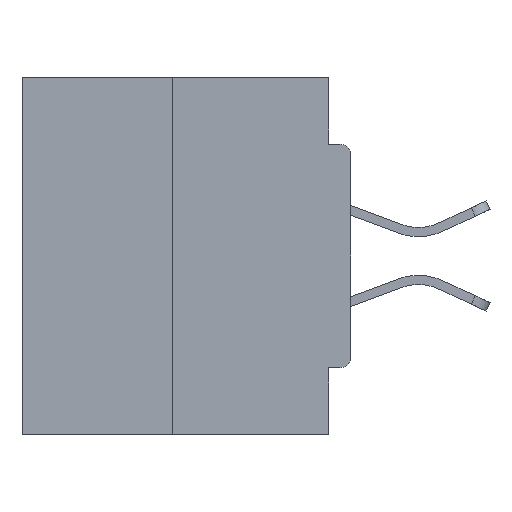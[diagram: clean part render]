
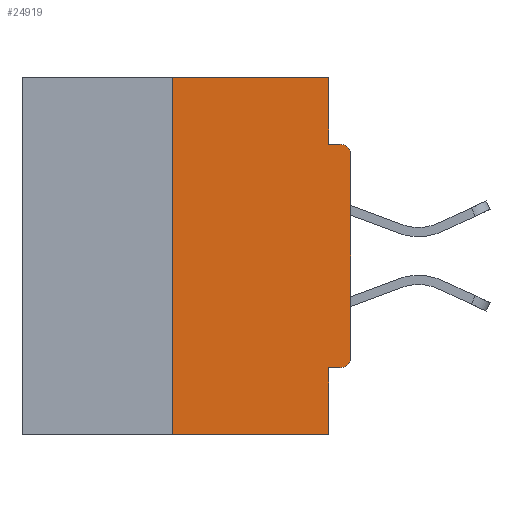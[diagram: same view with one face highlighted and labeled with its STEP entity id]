
A CAD part, left-side view. The second image highlights one B-rep face of the part: STEP entity #24919.
In plain terms, the highlighted planar face has unit normal (-1, 0, 0).
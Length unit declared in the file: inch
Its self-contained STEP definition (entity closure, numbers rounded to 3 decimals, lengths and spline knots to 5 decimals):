
#801 = EDGE_CURVE ( 'NONE', #25717, #2576, #8474, .T. ) ;
#1323 = LINE ( 'NONE', #11210, #20976 ) ;
#2336 = VERTEX_POINT ( 'NONE', #19962 ) ;
#2545 = CARTESIAN_POINT ( 'NONE',  ( 0., 0., 0. ) ) ;
#2576 = VERTEX_POINT ( 'NONE', #5639 ) ;
#3065 = AXIS2_PLACEMENT_3D ( 'NONE', #5719, #31607, #26658 ) ;
#4109 = DIRECTION ( 'NONE',  ( 0., 1., 0. ) ) ;
#4173 = VECTOR ( 'NONE', #32943, 39.37008 ) ;
#4766 = EDGE_CURVE ( 'NONE', #33345, #22715, #27988, .T. ) ;
#4966 = EDGE_CURVE ( 'NONE', #25717, #9873, #32548, .T. ) ;
#5000 = DIRECTION ( 'NONE',  ( 0., -1., 0. ) ) ;
#5095 = DIRECTION ( 'NONE',  ( 0., 0., 1. ) ) ;
#5639 = CARTESIAN_POINT ( 'NONE',  ( 0., 0., -0.3915 ) ) ;
#5697 = PLANE ( 'NONE',  #27454 ) ;
#5719 = CARTESIAN_POINT ( 'NONE',  ( 0., 0.015, -0.3915 ) ) ;
#5952 = VERTEX_POINT ( 'NONE', #12045 ) ;
#6232 = VECTOR ( 'NONE', #33441, 39.37008 ) ;
#7066 = LINE ( 'NONE', #14734, #4173 ) ;
#7301 = AXIS2_PLACEMENT_3D ( 'NONE', #10807, #23430, #23251 ) ;
#7408 = CARTESIAN_POINT ( 'NONE',  ( 0., 0.015, -0.0935 ) ) ;
#7714 = LINE ( 'NONE', #21163, #23079 ) ;
#8062 = EDGE_CURVE ( 'NONE', #2576, #2336, #18870, .T. ) ;
#8221 = DIRECTION ( 'NONE',  ( 0., 0., 1. ) ) ;
#8474 = CIRCLE ( 'NONE', #3065, 0.015 ) ;
#8845 = CARTESIAN_POINT ( 'NONE',  ( 0., 0.031, 0. ) ) ;
#9762 = LINE ( 'NONE', #28315, #9918 ) ;
#9873 = VERTEX_POINT ( 'NONE', #13396 ) ;
#9918 = VECTOR ( 'NONE', #12482, 39.37008 ) ;
#9944 = CARTESIAN_POINT ( 'NONE',  ( 0., 0.46, -0.5 ) ) ;
#10517 = EDGE_CURVE ( 'NONE', #5952, #23586, #12670, .T. ) ;
#10557 = CIRCLE ( 'NONE', #7301, 0.015 ) ;
#10807 = CARTESIAN_POINT ( 'NONE',  ( 0., 0.015, -0.1085 ) ) ;
#11210 = CARTESIAN_POINT ( 'NONE',  ( 0., 0.46, 0. ) ) ;
#11594 = EDGE_CURVE ( 'NONE', #20039, #13067, #1323, .T. ) ;
#11947 = CARTESIAN_POINT ( 'NONE',  ( 0., 0., -0.4065 ) ) ;
#12045 = CARTESIAN_POINT ( 'NONE',  ( 0., 0.031, -0.0935 ) ) ;
#12289 = ORIENTED_EDGE ( 'NONE', *, *, #14704, .F. ) ;
#12482 = DIRECTION ( 'NONE',  ( 0., 0., -1. ) ) ;
#12670 = LINE ( 'NONE', #33096, #6232 ) ;
#13067 = VERTEX_POINT ( 'NONE', #8845 ) ;
#13206 = DIRECTION ( 'NONE',  ( 1., 0., 0. ) ) ;
#13225 = ORIENTED_EDGE ( 'NONE', *, *, #4966, .F. ) ;
#13396 = CARTESIAN_POINT ( 'NONE',  ( 0., 0.031, -0.4065 ) ) ;
#14704 = EDGE_CURVE ( 'NONE', #13067, #5952, #7066, .T. ) ;
#14734 = CARTESIAN_POINT ( 'NONE',  ( 0., 0.031, 0. ) ) ;
#16136 = ORIENTED_EDGE ( 'NONE', *, *, #8062, .T. ) ;
#17710 = ORIENTED_EDGE ( 'NONE', *, *, #801, .T. ) ;
#18253 = ORIENTED_EDGE ( 'NONE', *, *, #20506, .F. ) ;
#18870 = LINE ( 'NONE', #2545, #24599 ) ;
#18982 = VECTOR ( 'NONE', #5000, 39.37008 ) ;
#19962 = CARTESIAN_POINT ( 'NONE',  ( 0., 0., -0.1085 ) ) ;
#20039 = VERTEX_POINT ( 'NONE', #29893 ) ;
#20506 = EDGE_CURVE ( 'NONE', #9873, #22715, #9762, .T. ) ;
#20778 = CARTESIAN_POINT ( 'NONE',  ( 0., 0.031, -0.5 ) ) ;
#20976 = VECTOR ( 'NONE', #29422, 39.37008 ) ;
#21163 = CARTESIAN_POINT ( 'NONE',  ( 0., 0.25, 0. ) ) ;
#21210 = CARTESIAN_POINT ( 'NONE',  ( 0., 0.46, 0. ) ) ;
#21585 = ORIENTED_EDGE ( 'NONE', *, *, #23635, .T. ) ;
#22715 = VERTEX_POINT ( 'NONE', #20778 ) ;
#23079 = VECTOR ( 'NONE', #8221, 39.37008 ) ;
#23170 = ORIENTED_EDGE ( 'NONE', *, *, #24106, .F. ) ;
#23251 = DIRECTION ( 'NONE',  ( 0., 0., -1. ) ) ;
#23430 = DIRECTION ( 'NONE',  ( -1., 0., 0. ) ) ;
#23586 = VERTEX_POINT ( 'NONE', #7408 ) ;
#23635 = EDGE_CURVE ( 'NONE', #2336, #23586, #10557, .T. ) ;
#24106 = EDGE_CURVE ( 'NONE', #33345, #20039, #7714, .T. ) ;
#24599 = VECTOR ( 'NONE', #5095, 39.37008 ) ;
#24719 = ORIENTED_EDGE ( 'NONE', *, *, #10517, .F. ) ;
#24919 = ADVANCED_FACE ( 'NONE', ( #26461 ), #5697, .F. ) ;
#25346 = CARTESIAN_POINT ( 'NONE',  ( 0., 0.25, -0.5 ) ) ;
#25717 = VERTEX_POINT ( 'NONE', #30658 ) ;
#25859 = ORIENTED_EDGE ( 'NONE', *, *, #11594, .F. ) ;
#26461 = FACE_OUTER_BOUND ( 'NONE', #33417, .T. ) ;
#26658 = DIRECTION ( 'NONE',  ( 0., 0., -1. ) ) ;
#27454 = AXIS2_PLACEMENT_3D ( 'NONE', #21210, #13206, #31583 ) ;
#27988 = LINE ( 'NONE', #9944, #18982 ) ;
#28315 = CARTESIAN_POINT ( 'NONE',  ( 0., 0.031, -0.5 ) ) ;
#29422 = DIRECTION ( 'NONE',  ( 0., -1., 0. ) ) ;
#29772 = ORIENTED_EDGE ( 'NONE', *, *, #4766, .T. ) ;
#29831 = VECTOR ( 'NONE', #4109, 39.37008 ) ;
#29893 = CARTESIAN_POINT ( 'NONE',  ( 0., 0.25, 0. ) ) ;
#30658 = CARTESIAN_POINT ( 'NONE',  ( 0., 0.015, -0.4065 ) ) ;
#31583 = DIRECTION ( 'NONE',  ( 0., 0., -1. ) ) ;
#31607 = DIRECTION ( 'NONE',  ( -1., 0., 0. ) ) ;
#32548 = LINE ( 'NONE', #11947, #29831 ) ;
#32943 = DIRECTION ( 'NONE',  ( 0., 0., -1. ) ) ;
#33096 = CARTESIAN_POINT ( 'NONE',  ( 0., 0., -0.0935 ) ) ;
#33345 = VERTEX_POINT ( 'NONE', #25346 ) ;
#33417 = EDGE_LOOP ( 'NONE', ( #25859, #23170, #29772, #18253, #13225, #17710, #16136, #21585, #24719, #12289 ) ) ;
#33441 = DIRECTION ( 'NONE',  ( 0., -1., 0. ) ) ;
